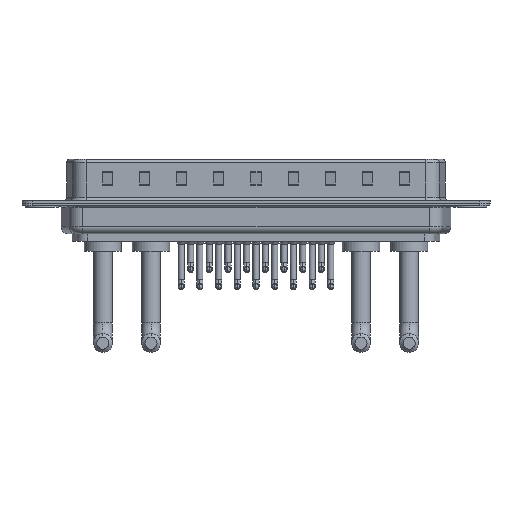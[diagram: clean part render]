
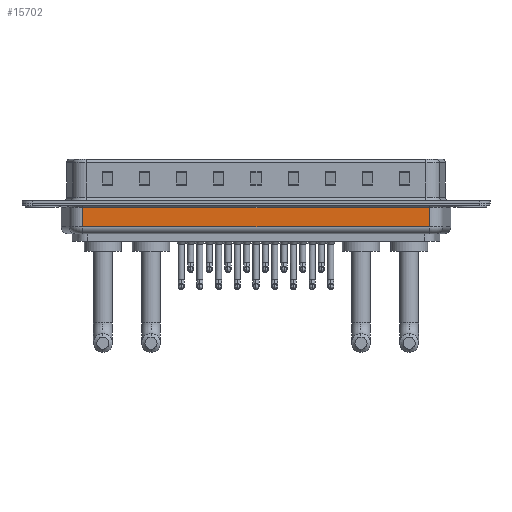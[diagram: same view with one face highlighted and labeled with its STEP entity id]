
A CAD part, front view. The second image highlights one B-rep face of the part: STEP entity #15702.
In plain terms, the highlighted planar face has unit normal (0, -1, 0).
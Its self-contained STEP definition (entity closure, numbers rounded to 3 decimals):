
#1618 = CARTESIAN_POINT ( 'NONE',  ( 57.469, -5.35, -4.5 ) ) ;
#2154 = CARTESIAN_POINT ( 'NONE',  ( 6.031, -5.35, -4.5 ) ) ;
#2171 = CARTESIAN_POINT ( 'NONE',  ( 6.031, -5.35, -4.5 ) ) ;
#2968 = VERTEX_POINT ( 'NONE', #16121 ) ;
#3231 = EDGE_CURVE ( 'NONE', #11212, #4292, #12850, .T. ) ;
#4049 = PLANE ( 'NONE',  #7663 ) ;
#4292 = VERTEX_POINT ( 'NONE', #8759 ) ;
#4318 = EDGE_CURVE ( 'NONE', #2968, #4292, #17296, .T. ) ;
#4900 = CARTESIAN_POINT ( 'NONE',  ( 6.031, -5.35, -0.65 ) ) ;
#6460 = EDGE_LOOP ( 'NONE', ( #22876, #19409, #7306, #23140 ) ) ;
#6901 = VECTOR ( 'NONE', #11643, 1000. ) ;
#7306 = ORIENTED_EDGE ( 'NONE', *, *, #8265, .T. ) ;
#7322 = DIRECTION ( 'NONE',  ( 0., 0., 1. ) ) ;
#7663 = AXIS2_PLACEMENT_3D ( 'NONE', #2154, #11886, #23626 ) ;
#8265 = EDGE_CURVE ( 'NONE', #10872, #11212, #20697, .T. ) ;
#8759 = CARTESIAN_POINT ( 'NONE',  ( 6.031, -5.35, -0.65 ) ) ;
#9039 = EDGE_CURVE ( 'NONE', #2968, #10872, #17051, .T. ) ;
#10872 = VERTEX_POINT ( 'NONE', #19795 ) ;
#11212 = VERTEX_POINT ( 'NONE', #15356 ) ;
#11643 = DIRECTION ( 'NONE',  ( 0., 0., 1. ) ) ;
#11886 = DIRECTION ( 'NONE',  ( 0., 1., 0. ) ) ;
#12850 = LINE ( 'NONE', #4900, #13308 ) ;
#13271 = CARTESIAN_POINT ( 'NONE',  ( 6.031, -5.35, -3.5 ) ) ;
#13308 = VECTOR ( 'NONE', #16987, 1000. ) ;
#15356 = CARTESIAN_POINT ( 'NONE',  ( 57.469, -5.35, -0.65 ) ) ;
#15702 = ADVANCED_FACE ( 'NONE', ( #21595 ), #4049, .F. ) ;
#16121 = CARTESIAN_POINT ( 'NONE',  ( 6.031, -5.35, -3.5 ) ) ;
#16987 = DIRECTION ( 'NONE',  ( -1., 0., 0. ) ) ;
#17051 = LINE ( 'NONE', #13271, #23890 ) ;
#17296 = LINE ( 'NONE', #2171, #6901 ) ;
#19409 = ORIENTED_EDGE ( 'NONE', *, *, #9039, .T. ) ;
#19795 = CARTESIAN_POINT ( 'NONE',  ( 57.469, -5.35, -3.5 ) ) ;
#20697 = LINE ( 'NONE', #1618, #21487 ) ;
#21487 = VECTOR ( 'NONE', #7322, 1000. ) ;
#21595 = FACE_OUTER_BOUND ( 'NONE', #6460, .T. ) ;
#22380 = DIRECTION ( 'NONE',  ( 1., 0., 0. ) ) ;
#22876 = ORIENTED_EDGE ( 'NONE', *, *, #4318, .F. ) ;
#23140 = ORIENTED_EDGE ( 'NONE', *, *, #3231, .T. ) ;
#23626 = DIRECTION ( 'NONE',  ( -1., 0., 0. ) ) ;
#23890 = VECTOR ( 'NONE', #22380, 1000. ) ;
